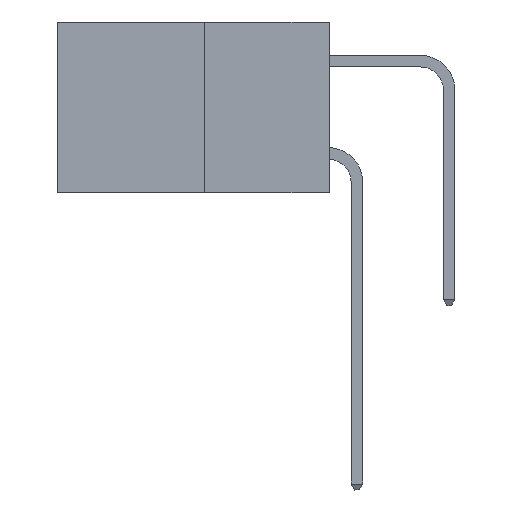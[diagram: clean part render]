
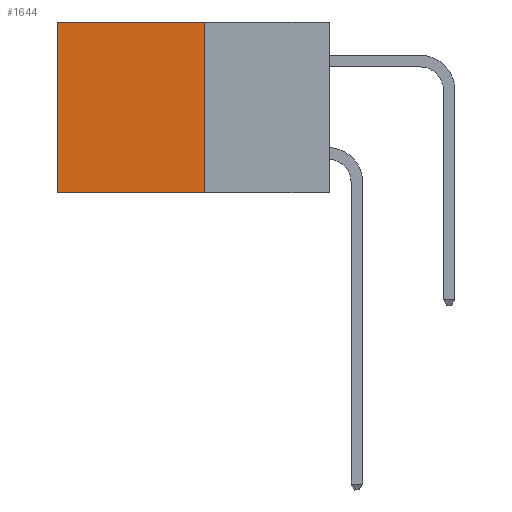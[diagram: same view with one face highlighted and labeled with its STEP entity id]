
A CAD part, left-side view. The second image highlights one B-rep face of the part: STEP entity #1644.
In plain terms, the highlighted planar face has unit normal (-1, 0, 0).
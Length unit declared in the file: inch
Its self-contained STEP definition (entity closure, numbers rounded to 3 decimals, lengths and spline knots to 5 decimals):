
#468 = VECTOR ( 'NONE', #3995, 39.37008 ) ;
#538 = DIRECTION ( 'NONE',  ( 0., 1., 0. ) ) ;
#1644 = ADVANCED_FACE ( 'NONE', ( #4278 ), #11892, .F. ) ;
#2710 = VERTEX_POINT ( 'NONE', #17828 ) ;
#3995 = DIRECTION ( 'NONE',  ( 0., 0., -1. ) ) ;
#4278 = FACE_OUTER_BOUND ( 'NONE', #17435, .T. ) ;
#4623 = CARTESIAN_POINT ( 'NONE',  ( 0.277, 0.59, -0.37 ) ) ;
#5013 = AXIS2_PLACEMENT_3D ( 'NONE', #15232, #11689, #15365 ) ;
#5372 = EDGE_CURVE ( 'NONE', #17975, #11904, #10861, .T. ) ;
#7173 = CARTESIAN_POINT ( 'NONE',  ( 0.277, 0.27, 0. ) ) ;
#7373 = CARTESIAN_POINT ( 'NONE',  ( 0.277, 0.59, -0.37 ) ) ;
#7519 = DIRECTION ( 'NONE',  ( 0., 0., -1. ) ) ;
#7759 = ORIENTED_EDGE ( 'NONE', *, *, #5372, .T. ) ;
#8749 = ORIENTED_EDGE ( 'NONE', *, *, #11546, .F. ) ;
#8851 = EDGE_CURVE ( 'NONE', #2710, #17975, #11041, .T. ) ;
#9693 = ORIENTED_EDGE ( 'NONE', *, *, #8851, .T. ) ;
#10155 = LINE ( 'NONE', #18209, #17484 ) ;
#10861 = LINE ( 'NONE', #7373, #18167 ) ;
#11041 = LINE ( 'NONE', #7173, #18341 ) ;
#11546 = EDGE_CURVE ( 'NONE', #2710, #11825, #15794, .T. ) ;
#11689 = DIRECTION ( 'NONE',  ( 1., 0., 0. ) ) ;
#11825 = VERTEX_POINT ( 'NONE', #16303 ) ;
#11892 = PLANE ( 'NONE',  #5013 ) ;
#11904 = VERTEX_POINT ( 'NONE', #4623 ) ;
#13362 = CARTESIAN_POINT ( 'NONE',  ( 0.277, 0.59, 0. ) ) ;
#15232 = CARTESIAN_POINT ( 'NONE',  ( 0.277, 0.27, -0.37 ) ) ;
#15365 = DIRECTION ( 'NONE',  ( 0., 0., -1. ) ) ;
#15794 = LINE ( 'NONE', #18600, #468 ) ;
#16216 = EDGE_CURVE ( 'NONE', #11825, #11904, #10155, .T. ) ;
#16303 = CARTESIAN_POINT ( 'NONE',  ( 0.277, 0.27, -0.37 ) ) ;
#17435 = EDGE_LOOP ( 'NONE', ( #7759, #17692, #8749, #9693 ) ) ;
#17484 = VECTOR ( 'NONE', #538, 39.37008 ) ;
#17692 = ORIENTED_EDGE ( 'NONE', *, *, #16216, .F. ) ;
#17828 = CARTESIAN_POINT ( 'NONE',  ( 0.277, 0.27, 0. ) ) ;
#17975 = VERTEX_POINT ( 'NONE', #13362 ) ;
#18167 = VECTOR ( 'NONE', #7519, 39.37008 ) ;
#18209 = CARTESIAN_POINT ( 'NONE',  ( 0.277, 0.27, -0.37 ) ) ;
#18341 = VECTOR ( 'NONE', #18862, 39.37008 ) ;
#18600 = CARTESIAN_POINT ( 'NONE',  ( 0.277, 0.27, -0.37 ) ) ;
#18862 = DIRECTION ( 'NONE',  ( 0., 1., 0. ) ) ;
